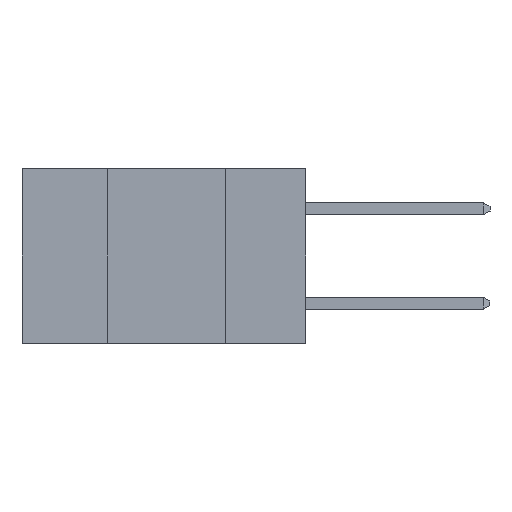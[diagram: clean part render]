
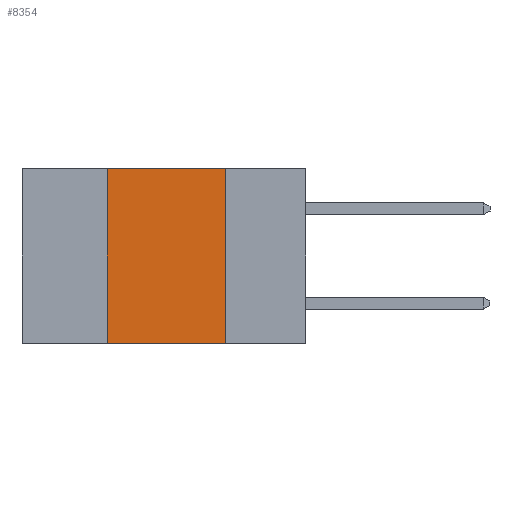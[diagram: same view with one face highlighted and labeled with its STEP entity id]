
A CAD part, left-side view. The second image highlights one B-rep face of the part: STEP entity #8354.
In plain terms, the highlighted planar face has unit normal (-1, 0, 0).
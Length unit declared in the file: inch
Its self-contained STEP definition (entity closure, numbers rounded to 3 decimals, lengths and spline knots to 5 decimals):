
#142 = EDGE_CURVE ( 'NONE', #12410, #10953, #13138, .T. ) ;
#942 = EDGE_CURVE ( 'NONE', #3994, #10953, #4084, .T. ) ;
#1771 = VECTOR ( 'NONE', #7985, 39.37008 ) ;
#1875 = EDGE_LOOP ( 'NONE', ( #9683, #12711, #5425, #11061 ) ) ;
#1908 = CARTESIAN_POINT ( 'NONE',  ( 0., 0.42, 0. ) ) ;
#2254 = PLANE ( 'NONE',  #8991 ) ;
#2273 = VECTOR ( 'NONE', #10453, 39.37008 ) ;
#3247 = DIRECTION ( 'NONE',  ( 0., 0., -1. ) ) ;
#3684 = CARTESIAN_POINT ( 'NONE',  ( 0., 0.17, -0.37 ) ) ;
#3796 = VECTOR ( 'NONE', #5511, 39.37008 ) ;
#3994 = VERTEX_POINT ( 'NONE', #9168 ) ;
#4084 = LINE ( 'NONE', #10901, #3796 ) ;
#5177 = CARTESIAN_POINT ( 'NONE',  ( 0., 0.6, 0. ) ) ;
#5305 = CARTESIAN_POINT ( 'NONE',  ( 0., 0.6, 0. ) ) ;
#5425 = ORIENTED_EDGE ( 'NONE', *, *, #8683, .F. ) ;
#5511 = DIRECTION ( 'NONE',  ( 0., -1., 0. ) ) ;
#7098 = LINE ( 'NONE', #1908, #1771 ) ;
#7355 = VERTEX_POINT ( 'NONE', #8846 ) ;
#7985 = DIRECTION ( 'NONE',  ( 0., 0., 1. ) ) ;
#8092 = VECTOR ( 'NONE', #12545, 39.37008 ) ;
#8354 = ADVANCED_FACE ( 'NONE', ( #11299 ), #2254, .F. ) ;
#8683 = EDGE_CURVE ( 'NONE', #3994, #7355, #7098, .T. ) ;
#8780 = CARTESIAN_POINT ( 'NONE',  ( 0., 0.17, 0. ) ) ;
#8846 = CARTESIAN_POINT ( 'NONE',  ( 0., 0.42, 0. ) ) ;
#8991 = AXIS2_PLACEMENT_3D ( 'NONE', #5177, #9390, #3247 ) ;
#9168 = CARTESIAN_POINT ( 'NONE',  ( 0., 0.42, -0.37 ) ) ;
#9390 = DIRECTION ( 'NONE',  ( 1., 0., 0. ) ) ;
#9529 = EDGE_CURVE ( 'NONE', #7355, #12410, #10819, .T. ) ;
#9683 = ORIENTED_EDGE ( 'NONE', *, *, #142, .F. ) ;
#10453 = DIRECTION ( 'NONE',  ( 0., 0., -1. ) ) ;
#10819 = LINE ( 'NONE', #5305, #8092 ) ;
#10901 = CARTESIAN_POINT ( 'NONE',  ( 0., 0.6, -0.37 ) ) ;
#10953 = VERTEX_POINT ( 'NONE', #3684 ) ;
#11061 = ORIENTED_EDGE ( 'NONE', *, *, #942, .T. ) ;
#11299 = FACE_OUTER_BOUND ( 'NONE', #1875, .T. ) ;
#12110 = CARTESIAN_POINT ( 'NONE',  ( 0., 0.17, 0. ) ) ;
#12410 = VERTEX_POINT ( 'NONE', #12110 ) ;
#12545 = DIRECTION ( 'NONE',  ( 0., -1., 0. ) ) ;
#12711 = ORIENTED_EDGE ( 'NONE', *, *, #9529, .F. ) ;
#13138 = LINE ( 'NONE', #8780, #2273 ) ;
